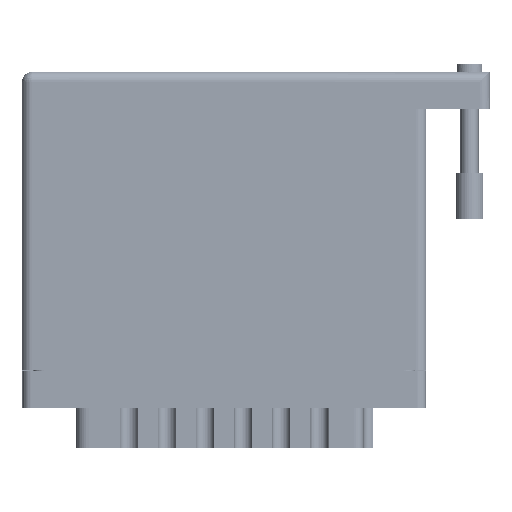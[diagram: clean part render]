
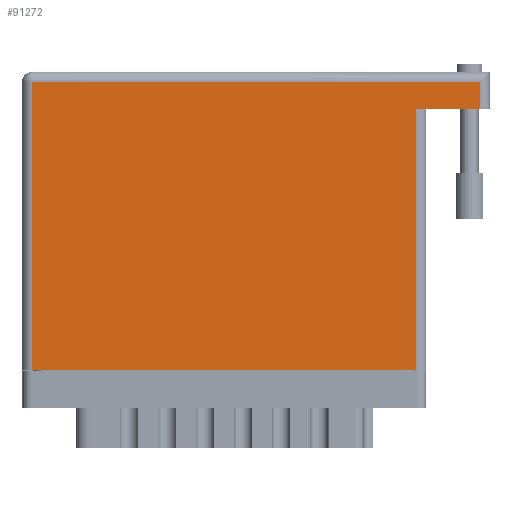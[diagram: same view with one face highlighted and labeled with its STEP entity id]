
A CAD part, front view. The second image highlights one B-rep face of the part: STEP entity #91272.
In plain terms, the highlighted face is planar.
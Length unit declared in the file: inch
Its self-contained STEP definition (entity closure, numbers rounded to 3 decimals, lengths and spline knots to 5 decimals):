
#5644 = LINE ( 'NONE', #72832, #79589 ) ;
#8565 = ORIENTED_EDGE ( 'NONE', *, *, #54439, .T. ) ;
#10415 = EDGE_CURVE ( 'NONE', #62350, #45547, #5644, .T. ) ;
#13517 = CARTESIAN_POINT ( 'NONE',  ( 0.07, 1.96, 0. ) ) ;
#15946 = ORIENTED_EDGE ( 'NONE', *, *, #92100, .F. ) ;
#15967 = VERTEX_POINT ( 'NONE', #47302 ) ;
#16916 = EDGE_CURVE ( 'NONE', #56606, #17798, #73951, .T. ) ;
#17675 = VECTOR ( 'NONE', #89968, 39.37008 ) ;
#17798 = VERTEX_POINT ( 'NONE', #13517 ) ;
#21659 = LINE ( 'NONE', #57642, #51918 ) ;
#24068 = ORIENTED_EDGE ( 'NONE', *, *, #10415, .T. ) ;
#24827 = DIRECTION ( 'NONE',  ( 0., 1., 0. ) ) ;
#24908 = CARTESIAN_POINT ( 'NONE',  ( 0., 0., 0. ) ) ;
#32944 = DIRECTION ( 'NONE',  ( -1., 0., 0. ) ) ;
#35226 = VECTOR ( 'NONE', #36271, 39.37008 ) ;
#36271 = DIRECTION ( 'NONE',  ( -1., 0., 0. ) ) ;
#39836 = CARTESIAN_POINT ( 'NONE',  ( 0., 2.03, 0. ) ) ;
#40067 = LINE ( 'NONE', #24908, #17675 ) ;
#41603 = VECTOR ( 'NONE', #24827, 39.37008 ) ;
#44273 = VERTEX_POINT ( 'NONE', #58934 ) ;
#45547 = VERTEX_POINT ( 'NONE', #52468 ) ;
#45706 = EDGE_CURVE ( 'NONE', #15967, #62350, #40067, .T. ) ;
#47302 = CARTESIAN_POINT ( 'NONE',  ( 0.07, 0., 0. ) ) ;
#48703 = EDGE_CURVE ( 'NONE', #17798, #15967, #21659, .T. ) ;
#50836 = ORIENTED_EDGE ( 'NONE', *, *, #48703, .T. ) ;
#51337 = ORIENTED_EDGE ( 'NONE', *, *, #45706, .T. ) ;
#51918 = VECTOR ( 'NONE', #86705, 39.37008 ) ;
#52468 = CARTESIAN_POINT ( 'NONE',  ( 2.685, 1.774, 0. ) ) ;
#53599 = CARTESIAN_POINT ( 'NONE',  ( 3.12, 1.96, 0. ) ) ;
#54439 = EDGE_CURVE ( 'NONE', #44273, #56606, #81870, .T. ) ;
#56606 = VERTEX_POINT ( 'NONE', #53599 ) ;
#57642 = CARTESIAN_POINT ( 'NONE',  ( 0.07, 0., 0. ) ) ;
#58934 = CARTESIAN_POINT ( 'NONE',  ( 3.12, 1.774, 0. ) ) ;
#59450 = ORIENTED_EDGE ( 'NONE', *, *, #16916, .T. ) ;
#62350 = VERTEX_POINT ( 'NONE', #67993 ) ;
#67650 = AXIS2_PLACEMENT_3D ( 'NONE', #39836, #82040, #32944 ) ;
#67670 = CARTESIAN_POINT ( 'NONE',  ( 3.12, 2.03, 0. ) ) ;
#67993 = CARTESIAN_POINT ( 'NONE',  ( 2.685, 0., 0. ) ) ;
#68877 = CARTESIAN_POINT ( 'NONE',  ( 0., 1.96, 0. ) ) ;
#69496 = DIRECTION ( 'NONE',  ( -1., 0., 0. ) ) ;
#71017 = LINE ( 'NONE', #71308, #35226 ) ;
#71308 = CARTESIAN_POINT ( 'NONE',  ( 3.19, 1.774, 0. ) ) ;
#72832 = CARTESIAN_POINT ( 'NONE',  ( 2.685, 1.774, 0. ) ) ;
#72844 = VECTOR ( 'NONE', #69496, 39.37008 ) ;
#73951 = LINE ( 'NONE', #68877, #72844 ) ;
#74081 = DIRECTION ( 'NONE',  ( 0., 1., 0. ) ) ;
#76108 = PLANE ( 'NONE',  #67650 ) ;
#79589 = VECTOR ( 'NONE', #74081, 39.37008 ) ;
#80035 = FACE_OUTER_BOUND ( 'NONE', #88267, .T. ) ;
#81870 = LINE ( 'NONE', #67670, #41603 ) ;
#82040 = DIRECTION ( 'NONE',  ( 0., 0., -1. ) ) ;
#86705 = DIRECTION ( 'NONE',  ( 0., -1., 0. ) ) ;
#88267 = EDGE_LOOP ( 'NONE', ( #51337, #24068, #15946, #8565, #59450, #50836 ) ) ;
#89968 = DIRECTION ( 'NONE',  ( 1., 0., 0. ) ) ;
#91272 = ADVANCED_FACE ( 'NONE', ( #80035 ), #76108, .F. ) ;
#92100 = EDGE_CURVE ( 'NONE', #44273, #45547, #71017, .T. ) ;
